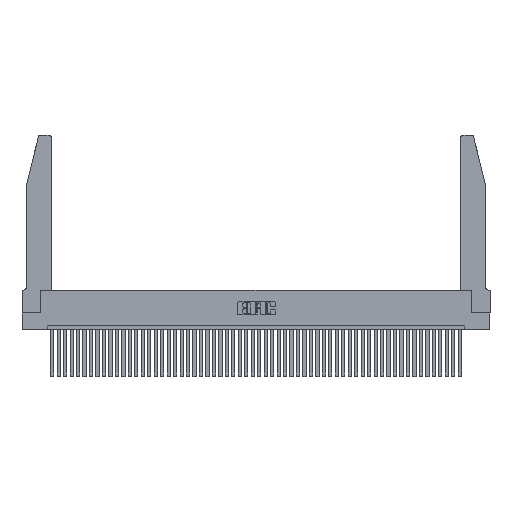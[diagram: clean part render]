
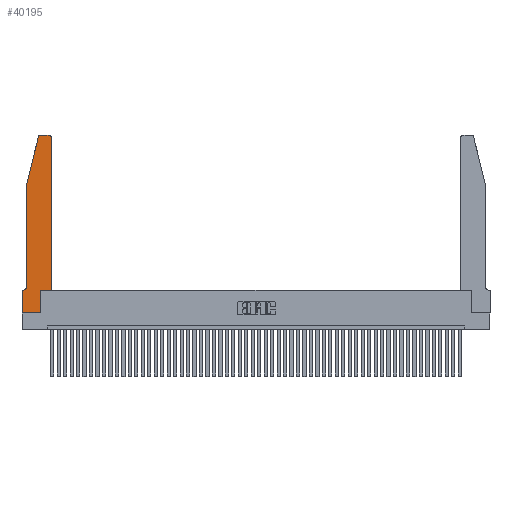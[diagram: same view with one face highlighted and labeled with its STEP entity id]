
A CAD part, top view. The second image highlights one B-rep face of the part: STEP entity #40195.
In plain terms, the highlighted planar face has unit normal (0, 0, 1).
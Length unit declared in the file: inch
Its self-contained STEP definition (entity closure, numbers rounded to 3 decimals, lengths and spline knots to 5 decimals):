
#778 = AXIS2_PLACEMENT_3D ( 'NONE', #13199, #40053, #5644 ) ;
#953 = CARTESIAN_POINT ( 'NONE',  ( 0.2605, 2.75, 0.37 ) ) ;
#1157 = VERTEX_POINT ( 'NONE', #45861 ) ;
#1459 = LINE ( 'NONE', #23938, #38658 ) ;
#2307 = VERTEX_POINT ( 'NONE', #44223 ) ;
#2476 = ORIENTED_EDGE ( 'NONE', *, *, #6438, .T. ) ;
#2819 = VERTEX_POINT ( 'NONE', #13032 ) ;
#3193 = EDGE_CURVE ( 'NONE', #1157, #45760, #20416, .T. ) ;
#4258 = CARTESIAN_POINT ( 'NONE',  ( 0.4205, 2.72, 0.37 ) ) ;
#4688 = CARTESIAN_POINT ( 'NONE',  ( 0.0755, 2., 0.37 ) ) ;
#5025 = VERTEX_POINT ( 'NONE', #34142 ) ;
#5042 = LINE ( 'NONE', #27617, #44728 ) ;
#5644 = DIRECTION ( 'NONE',  ( 1., 0., 0. ) ) ;
#5682 = DIRECTION ( 'NONE',  ( 0., -1., 0. ) ) ;
#5980 = DIRECTION ( 'NONE',  ( 0., -1., 0. ) ) ;
#6160 = VERTEX_POINT ( 'NONE', #40796 ) ;
#6438 = EDGE_CURVE ( 'NONE', #2819, #35825, #5042, .T. ) ;
#6931 = ORIENTED_EDGE ( 'NONE', *, *, #38681, .T. ) ;
#8682 = CARTESIAN_POINT ( 'NONE',  ( 0.0755, 2., 0.37 ) ) ;
#8780 = CARTESIAN_POINT ( 'NONE',  ( 0.4505, 0.35, 0.37 ) ) ;
#9035 = VECTOR ( 'NONE', #22481, 39.37008 ) ;
#9683 = CARTESIAN_POINT ( 'NONE',  ( 0., 0., 0.37 ) ) ;
#10190 = EDGE_CURVE ( 'NONE', #6160, #26204, #34117, .T. ) ;
#11122 = ORIENTED_EDGE ( 'NONE', *, *, #30362, .T. ) ;
#11585 = CIRCLE ( 'NONE', #27383, 0.03 ) ;
#13032 = CARTESIAN_POINT ( 'NONE',  ( 0.2865, 0.35, 0.37 ) ) ;
#13199 = CARTESIAN_POINT ( 'NONE',  ( 0.284, 2.72, 0.37 ) ) ;
#13218 = CARTESIAN_POINT ( 'NONE',  ( 0., 0.35, 0.37 ) ) ;
#13815 = CARTESIAN_POINT ( 'NONE',  ( 0.4505, 0.35, 0.37 ) ) ;
#13993 = LINE ( 'NONE', #36351, #17011 ) ;
#15182 = DIRECTION ( 'NONE',  ( 0., 0., 1. ) ) ;
#16283 = ORIENTED_EDGE ( 'NONE', *, *, #44985, .T. ) ;
#17011 = VECTOR ( 'NONE', #28144, 39.37008 ) ;
#17571 = LINE ( 'NONE', #24131, #33183 ) ;
#18121 = CARTESIAN_POINT ( 'NONE',  ( 0.0755, 0.35, 0.37 ) ) ;
#18584 = EDGE_CURVE ( 'NONE', #38554, #5025, #17571, .T. ) ;
#18594 = EDGE_CURVE ( 'NONE', #2307, #2819, #13993, .T. ) ;
#18944 = ORIENTED_EDGE ( 'NONE', *, *, #10190, .T. ) ;
#19037 = ORIENTED_EDGE ( 'NONE', *, *, #32366, .T. ) ;
#19229 = DIRECTION ( 'NONE',  ( 0., 0., 1. ) ) ;
#19564 = DIRECTION ( 'NONE',  ( 1., 0., 0. ) ) ;
#20416 = LINE ( 'NONE', #18121, #9035 ) ;
#22239 = VECTOR ( 'NONE', #5980, 39.37008 ) ;
#22481 = DIRECTION ( 'NONE',  ( -1., 0., 0. ) ) ;
#23512 = CIRCLE ( 'NONE', #778, 0.03 ) ;
#23580 = VECTOR ( 'NONE', #38581, 39.37008 ) ;
#23938 = CARTESIAN_POINT ( 'NONE',  ( 0., 0., 0.37 ) ) ;
#23969 = CARTESIAN_POINT ( 'NONE',  ( 0., 0., 0.37 ) ) ;
#24131 = CARTESIAN_POINT ( 'NONE',  ( 0.0755, 2., 0.37 ) ) ;
#24182 = VECTOR ( 'NONE', #48428, 39.37008 ) ;
#26204 = VERTEX_POINT ( 'NONE', #41730 ) ;
#26860 = CARTESIAN_POINT ( 'NONE',  ( 0.0055, 0.42, 0.37 ) ) ;
#27383 = AXIS2_PLACEMENT_3D ( 'NONE', #4258, #15182, #42042 ) ;
#27617 = CARTESIAN_POINT ( 'NONE',  ( 0.4505, 0.35, 0.37 ) ) ;
#28144 = DIRECTION ( 'NONE',  ( 0., 1., 0. ) ) ;
#29700 = EDGE_CURVE ( 'NONE', #43167, #2307, #1459, .T. ) ;
#29899 = FACE_OUTER_BOUND ( 'NONE', #48500, .T. ) ;
#30362 = EDGE_CURVE ( 'NONE', #45855, #6160, #11585, .T. ) ;
#31293 = DIRECTION ( 'NONE',  ( 1., 0., 0. ) ) ;
#31311 = ORIENTED_EDGE ( 'NONE', *, *, #29700, .T. ) ;
#31631 = DIRECTION ( 'NONE',  ( -1., 0., 0. ) ) ;
#31967 = ORIENTED_EDGE ( 'NONE', *, *, #3193, .T. ) ;
#32366 = EDGE_CURVE ( 'NONE', #26204, #49372, #23512, .T. ) ;
#33183 = VECTOR ( 'NONE', #5682, 39.37008 ) ;
#33241 = EDGE_CURVE ( 'NONE', #5025, #1157, #49274, .T. ) ;
#34117 = LINE ( 'NONE', #953, #48016 ) ;
#34142 = CARTESIAN_POINT ( 'NONE',  ( 0.0755, 0.42, 0.37 ) ) ;
#34356 = PLANE ( 'NONE',  #38427 ) ;
#34509 = DIRECTION ( 'NONE',  ( 1., 0., 0. ) ) ;
#34976 = LINE ( 'NONE', #4688, #23580 ) ;
#35825 = VERTEX_POINT ( 'NONE', #8780 ) ;
#36351 = CARTESIAN_POINT ( 'NONE',  ( 0.2865, 0.35, 0.37 ) ) ;
#37254 = DIRECTION ( 'NONE',  ( -1., 0., 0. ) ) ;
#37344 = EDGE_CURVE ( 'NONE', #35825, #45855, #45865, .T. ) ;
#38121 = ORIENTED_EDGE ( 'NONE', *, *, #33241, .T. ) ;
#38427 = AXIS2_PLACEMENT_3D ( 'NONE', #38869, #19229, #34509 ) ;
#38554 = VERTEX_POINT ( 'NONE', #8682 ) ;
#38575 = CARTESIAN_POINT ( 'NONE',  ( 0.25487, 2.72718, 0.37 ) ) ;
#38581 = DIRECTION ( 'NONE',  ( -0.239, -0.971, 0. ) ) ;
#38658 = VECTOR ( 'NONE', #19564, 39.37008 ) ;
#38681 = EDGE_CURVE ( 'NONE', #45760, #43167, #42069, .T. ) ;
#38869 = CARTESIAN_POINT ( 'NONE',  ( 0., 0.35, 0.37 ) ) ;
#39509 = ORIENTED_EDGE ( 'NONE', *, *, #37344, .T. ) ;
#39909 = CARTESIAN_POINT ( 'NONE',  ( 0.4505, 2.72, 0.37 ) ) ;
#40053 = DIRECTION ( 'NONE',  ( 0., 0., 1. ) ) ;
#40195 = ADVANCED_FACE ( 'NONE', ( #29899 ), #34356, .T. ) ;
#40660 = ORIENTED_EDGE ( 'NONE', *, *, #18594, .T. ) ;
#40796 = CARTESIAN_POINT ( 'NONE',  ( 0.4205, 2.75, 0.37 ) ) ;
#41730 = CARTESIAN_POINT ( 'NONE',  ( 0.284, 2.75, 0.37 ) ) ;
#42042 = DIRECTION ( 'NONE',  ( 1., 0., 0. ) ) ;
#42069 = LINE ( 'NONE', #9683, #22239 ) ;
#43167 = VERTEX_POINT ( 'NONE', #23969 ) ;
#44223 = CARTESIAN_POINT ( 'NONE',  ( 0.2865, 0., 0.37 ) ) ;
#44728 = VECTOR ( 'NONE', #31293, 39.37008 ) ;
#44793 = ORIENTED_EDGE ( 'NONE', *, *, #18584, .T. ) ;
#44985 = EDGE_CURVE ( 'NONE', #49372, #38554, #34976, .T. ) ;
#45052 = DIRECTION ( 'NONE',  ( 0., 0., -1. ) ) ;
#45760 = VERTEX_POINT ( 'NONE', #13218 ) ;
#45855 = VERTEX_POINT ( 'NONE', #39909 ) ;
#45861 = CARTESIAN_POINT ( 'NONE',  ( 0.0055, 0.35, 0.37 ) ) ;
#45865 = LINE ( 'NONE', #13815, #24182 ) ;
#48016 = VECTOR ( 'NONE', #31631, 39.37008 ) ;
#48428 = DIRECTION ( 'NONE',  ( 0., 1., 0. ) ) ;
#48500 = EDGE_LOOP ( 'NONE', ( #18944, #19037, #16283, #44793, #38121, #31967, #6931, #31311, #40660, #2476, #39509, #11122 ) ) ;
#48764 = AXIS2_PLACEMENT_3D ( 'NONE', #26860, #45052, #37254 ) ;
#49274 = CIRCLE ( 'NONE', #48764, 0.07 ) ;
#49372 = VERTEX_POINT ( 'NONE', #38575 ) ;
